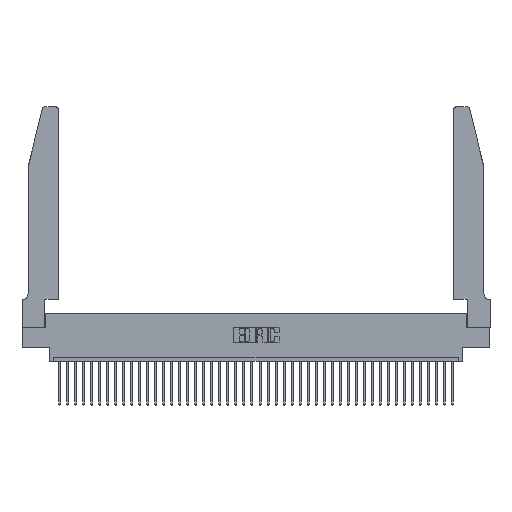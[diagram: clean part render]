
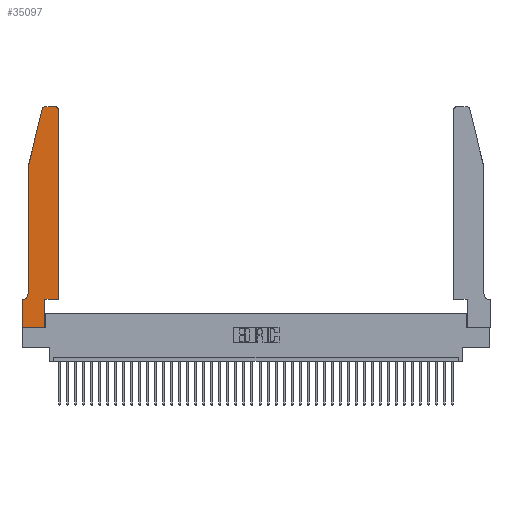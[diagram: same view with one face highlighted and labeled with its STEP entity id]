
A CAD part, top view. The second image highlights one B-rep face of the part: STEP entity #35097.
In plain terms, the highlighted planar face has unit normal (0, 0, 1).
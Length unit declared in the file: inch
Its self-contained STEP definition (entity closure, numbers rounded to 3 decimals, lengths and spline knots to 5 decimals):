
#564 = LINE ( 'NONE', #6837, #39104 ) ;
#1544 = CARTESIAN_POINT ( 'NONE',  ( 0.2865, 0.35, 0.37 ) ) ;
#1696 = EDGE_CURVE ( 'NONE', #13420, #16253, #11762, .T. ) ;
#1704 = VERTEX_POINT ( 'NONE', #27631 ) ;
#1741 = ORIENTED_EDGE ( 'NONE', *, *, #12218, .T. ) ;
#1919 = CARTESIAN_POINT ( 'NONE',  ( 0.284, 2.72, 0.37 ) ) ;
#3001 = EDGE_CURVE ( 'NONE', #29167, #19016, #7085, .T. ) ;
#3295 = DIRECTION ( 'NONE',  ( 1., 0., 0. ) ) ;
#3308 = LINE ( 'NONE', #8215, #20735 ) ;
#3551 = PLANE ( 'NONE',  #12472 ) ;
#3709 = VERTEX_POINT ( 'NONE', #22518 ) ;
#3761 = ORIENTED_EDGE ( 'NONE', *, *, #1696, .T. ) ;
#4050 = DIRECTION ( 'NONE',  ( 0., 1., 0. ) ) ;
#5666 = CARTESIAN_POINT ( 'NONE',  ( 0.0755, 2., 0.37 ) ) ;
#5930 = LINE ( 'NONE', #20801, #14310 ) ;
#6373 = AXIS2_PLACEMENT_3D ( 'NONE', #25146, #9091, #18270 ) ;
#6837 = CARTESIAN_POINT ( 'NONE',  ( 0.2865, 0.35, 0.37 ) ) ;
#7085 = LINE ( 'NONE', #12276, #29130 ) ;
#8068 = CARTESIAN_POINT ( 'NONE',  ( 0.4505, 0.35, 0.37 ) ) ;
#8215 = CARTESIAN_POINT ( 'NONE',  ( 0.0755, 2., 0.37 ) ) ;
#9091 = DIRECTION ( 'NONE',  ( 0., 0., -1. ) ) ;
#9218 = VERTEX_POINT ( 'NONE', #8068 ) ;
#9555 = VECTOR ( 'NONE', #23310, 39.37008 ) ;
#9753 = CARTESIAN_POINT ( 'NONE',  ( 0.284, 2.75, 0.37 ) ) ;
#9795 = DIRECTION ( 'NONE',  ( 0., -1., 0. ) ) ;
#9985 = ORIENTED_EDGE ( 'NONE', *, *, #31444, .T. ) ;
#10015 = EDGE_CURVE ( 'NONE', #27828, #28177, #25625, .T. ) ;
#10258 = CARTESIAN_POINT ( 'NONE',  ( 0.4205, 2.72, 0.37 ) ) ;
#11203 = LINE ( 'NONE', #38717, #35258 ) ;
#11762 = LINE ( 'NONE', #30705, #26700 ) ;
#12218 = EDGE_CURVE ( 'NONE', #37446, #29167, #14983, .T. ) ;
#12276 = CARTESIAN_POINT ( 'NONE',  ( 0., 0., 0.37 ) ) ;
#12472 = AXIS2_PLACEMENT_3D ( 'NONE', #35414, #38400, #3295 ) ;
#13420 = VERTEX_POINT ( 'NONE', #5666 ) ;
#13661 = EDGE_CURVE ( 'NONE', #1704, #37446, #23251, .T. ) ;
#14310 = VECTOR ( 'NONE', #27587, 39.37008 ) ;
#14696 = ORIENTED_EDGE ( 'NONE', *, *, #38603, .T. ) ;
#14983 = LINE ( 'NONE', #18884, #38041 ) ;
#15371 = ORIENTED_EDGE ( 'NONE', *, *, #30781, .T. ) ;
#16253 = VERTEX_POINT ( 'NONE', #21472 ) ;
#17105 = CARTESIAN_POINT ( 'NONE',  ( 0., 0.35, 0.37 ) ) ;
#17634 = DIRECTION ( 'NONE',  ( 0., -1., 0. ) ) ;
#18130 = EDGE_CURVE ( 'NONE', #16253, #1704, #29760, .T. ) ;
#18233 = CARTESIAN_POINT ( 'NONE',  ( 0.25487, 2.72718, 0.37 ) ) ;
#18270 = DIRECTION ( 'NONE',  ( -1., 0., 0. ) ) ;
#18884 = CARTESIAN_POINT ( 'NONE',  ( 0., 0., 0.37 ) ) ;
#19016 = VERTEX_POINT ( 'NONE', #23485 ) ;
#19797 = VERTEX_POINT ( 'NONE', #1544 ) ;
#20279 = AXIS2_PLACEMENT_3D ( 'NONE', #10258, #38950, #35850 ) ;
#20606 = EDGE_CURVE ( 'NONE', #19016, #19797, #564, .T. ) ;
#20735 = VECTOR ( 'NONE', #37323, 39.37008 ) ;
#20801 = CARTESIAN_POINT ( 'NONE',  ( 0.2605, 2.75, 0.37 ) ) ;
#21472 = CARTESIAN_POINT ( 'NONE',  ( 0.0755, 0.42, 0.37 ) ) ;
#21620 = DIRECTION ( 'NONE',  ( 1., 0., 0. ) ) ;
#22518 = CARTESIAN_POINT ( 'NONE',  ( 0.4505, 2.72, 0.37 ) ) ;
#23251 = LINE ( 'NONE', #40367, #29824 ) ;
#23310 = DIRECTION ( 'NONE',  ( 1., 0., 0. ) ) ;
#23316 = EDGE_CURVE ( 'NONE', #3709, #40473, #37504, .T. ) ;
#23485 = CARTESIAN_POINT ( 'NONE',  ( 0.2865, 0., 0.37 ) ) ;
#23741 = CARTESIAN_POINT ( 'NONE',  ( 0., 0., 0.37 ) ) ;
#23878 = ORIENTED_EDGE ( 'NONE', *, *, #13661, .T. ) ;
#24650 = DIRECTION ( 'NONE',  ( -1., 0., 0. ) ) ;
#25146 = CARTESIAN_POINT ( 'NONE',  ( 0.0055, 0.42, 0.37 ) ) ;
#25625 = CIRCLE ( 'NONE', #36085, 0.03 ) ;
#26535 = FACE_OUTER_BOUND ( 'NONE', #33208, .T. ) ;
#26700 = VECTOR ( 'NONE', #17634, 39.37008 ) ;
#27587 = DIRECTION ( 'NONE',  ( -1., 0., 0. ) ) ;
#27631 = CARTESIAN_POINT ( 'NONE',  ( 0.0055, 0.35, 0.37 ) ) ;
#27828 = VERTEX_POINT ( 'NONE', #9753 ) ;
#28177 = VERTEX_POINT ( 'NONE', #18233 ) ;
#28404 = EDGE_CURVE ( 'NONE', #19797, #9218, #31096, .T. ) ;
#28878 = ORIENTED_EDGE ( 'NONE', *, *, #28404, .T. ) ;
#28939 = ORIENTED_EDGE ( 'NONE', *, *, #23316, .T. ) ;
#29084 = ORIENTED_EDGE ( 'NONE', *, *, #10015, .T. ) ;
#29130 = VECTOR ( 'NONE', #21620, 39.37008 ) ;
#29167 = VERTEX_POINT ( 'NONE', #23741 ) ;
#29760 = CIRCLE ( 'NONE', #6373, 0.07 ) ;
#29824 = VECTOR ( 'NONE', #24650, 39.37008 ) ;
#29911 = DIRECTION ( 'NONE',  ( 1., 0., 0. ) ) ;
#30021 = ORIENTED_EDGE ( 'NONE', *, *, #3001, .T. ) ;
#30705 = CARTESIAN_POINT ( 'NONE',  ( 0.0755, 2., 0.37 ) ) ;
#30781 = EDGE_CURVE ( 'NONE', #40473, #27828, #5930, .T. ) ;
#31096 = LINE ( 'NONE', #36109, #9555 ) ;
#31444 = EDGE_CURVE ( 'NONE', #28177, #13420, #3308, .T. ) ;
#32992 = DIRECTION ( 'NONE',  ( 0., 0., 1. ) ) ;
#33208 = EDGE_LOOP ( 'NONE', ( #15371, #29084, #9985, #3761, #35189, #23878, #1741, #30021, #38915, #28878, #14696, #28939 ) ) ;
#35097 = ADVANCED_FACE ( 'NONE', ( #26535 ), #3551, .T. ) ;
#35189 = ORIENTED_EDGE ( 'NONE', *, *, #18130, .T. ) ;
#35258 = VECTOR ( 'NONE', #38591, 39.37008 ) ;
#35414 = CARTESIAN_POINT ( 'NONE',  ( 0., 0.35, 0.37 ) ) ;
#35850 = DIRECTION ( 'NONE',  ( 1., 0., 0. ) ) ;
#36085 = AXIS2_PLACEMENT_3D ( 'NONE', #1919, #32992, #29911 ) ;
#36109 = CARTESIAN_POINT ( 'NONE',  ( 0.4505, 0.35, 0.37 ) ) ;
#37323 = DIRECTION ( 'NONE',  ( -0.239, -0.971, 0. ) ) ;
#37446 = VERTEX_POINT ( 'NONE', #17105 ) ;
#37504 = CIRCLE ( 'NONE', #20279, 0.03 ) ;
#38041 = VECTOR ( 'NONE', #9795, 39.37008 ) ;
#38400 = DIRECTION ( 'NONE',  ( 0., 0., 1. ) ) ;
#38591 = DIRECTION ( 'NONE',  ( 0., 1., 0. ) ) ;
#38603 = EDGE_CURVE ( 'NONE', #9218, #3709, #11203, .T. ) ;
#38717 = CARTESIAN_POINT ( 'NONE',  ( 0.4505, 0.35, 0.37 ) ) ;
#38915 = ORIENTED_EDGE ( 'NONE', *, *, #20606, .T. ) ;
#38950 = DIRECTION ( 'NONE',  ( 0., 0., 1. ) ) ;
#39104 = VECTOR ( 'NONE', #4050, 39.37008 ) ;
#40092 = CARTESIAN_POINT ( 'NONE',  ( 0.4205, 2.75, 0.37 ) ) ;
#40367 = CARTESIAN_POINT ( 'NONE',  ( 0.0755, 0.35, 0.37 ) ) ;
#40473 = VERTEX_POINT ( 'NONE', #40092 ) ;
